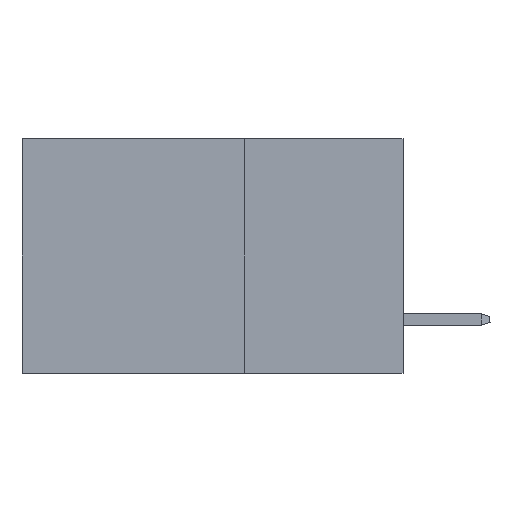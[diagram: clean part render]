
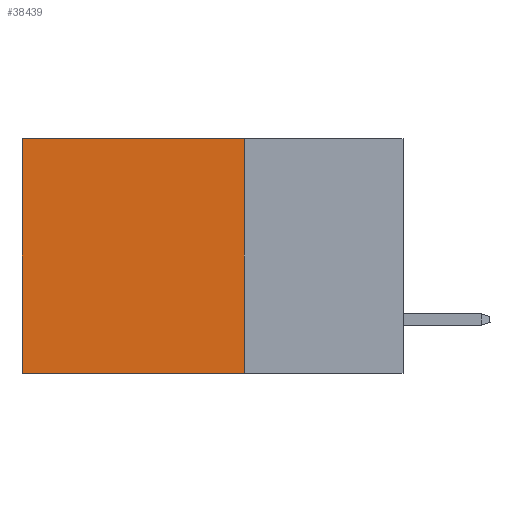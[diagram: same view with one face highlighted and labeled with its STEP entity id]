
A CAD part, left-side view. The second image highlights one B-rep face of the part: STEP entity #38439.
In plain terms, the highlighted planar face has unit normal (-1, 0, 0).
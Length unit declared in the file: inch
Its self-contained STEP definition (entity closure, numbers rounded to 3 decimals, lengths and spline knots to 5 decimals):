
#298 = EDGE_CURVE ( 'NONE', #982, #2464, #387, .T. ) ;
#365 = ORIENTED_EDGE ( 'NONE', *, *, #30370, .T. ) ;
#387 = LINE ( 'NONE', #4774, #18558 ) ;
#982 = VERTEX_POINT ( 'NONE', #10057 ) ;
#2464 = VERTEX_POINT ( 'NONE', #10327 ) ;
#2769 = PLANE ( 'NONE',  #32725 ) ;
#4774 = CARTESIAN_POINT ( 'NONE',  ( 0.2875, 0.25, -0.37 ) ) ;
#5797 = EDGE_LOOP ( 'NONE', ( #17149, #30770, #29971, #365 ) ) ;
#7968 = DIRECTION ( 'NONE',  ( 0., 1., 0. ) ) ;
#8990 = VERTEX_POINT ( 'NONE', #40663 ) ;
#10057 = CARTESIAN_POINT ( 'NONE',  ( 0.2875, 0.25, -0.37 ) ) ;
#10327 = CARTESIAN_POINT ( 'NONE',  ( 0.2875, 0.6, -0.37 ) ) ;
#11798 = DIRECTION ( 'NONE',  ( 0., 0., -1. ) ) ;
#12013 = CARTESIAN_POINT ( 'NONE',  ( 0.2875, 0.25, 0. ) ) ;
#12520 = VECTOR ( 'NONE', #30075, 39.37008 ) ;
#17149 = ORIENTED_EDGE ( 'NONE', *, *, #37518, .T. ) ;
#18558 = VECTOR ( 'NONE', #7968, 39.37008 ) ;
#18881 = CARTESIAN_POINT ( 'NONE',  ( 0.2875, 0.6, 0. ) ) ;
#19336 = LINE ( 'NONE', #12013, #43485 ) ;
#19442 = EDGE_CURVE ( 'NONE', #45630, #982, #19336, .T. ) ;
#22244 = CARTESIAN_POINT ( 'NONE',  ( 0.2875, 0.25, 0. ) ) ;
#26470 = LINE ( 'NONE', #18881, #32688 ) ;
#28960 = CARTESIAN_POINT ( 'NONE',  ( 0.2875, 0.25, 0. ) ) ;
#29971 = ORIENTED_EDGE ( 'NONE', *, *, #19442, .F. ) ;
#30075 = DIRECTION ( 'NONE',  ( 0., 1., 0. ) ) ;
#30370 = EDGE_CURVE ( 'NONE', #45630, #8990, #37413, .T. ) ;
#30770 = ORIENTED_EDGE ( 'NONE', *, *, #298, .F. ) ;
#30841 = DIRECTION ( 'NONE',  ( 0., 0., -1. ) ) ;
#31642 = CARTESIAN_POINT ( 'NONE',  ( 0.2875, 0.25, 0. ) ) ;
#32688 = VECTOR ( 'NONE', #11798, 39.37008 ) ;
#32725 = AXIS2_PLACEMENT_3D ( 'NONE', #31642, #43374, #39706 ) ;
#37413 = LINE ( 'NONE', #22244, #12520 ) ;
#37518 = EDGE_CURVE ( 'NONE', #8990, #2464, #26470, .T. ) ;
#38439 = ADVANCED_FACE ( 'NONE', ( #43607 ), #2769, .F. ) ;
#39706 = DIRECTION ( 'NONE',  ( 0., 0., -1. ) ) ;
#40663 = CARTESIAN_POINT ( 'NONE',  ( 0.2875, 0.6, 0. ) ) ;
#43374 = DIRECTION ( 'NONE',  ( 1., 0., 0. ) ) ;
#43485 = VECTOR ( 'NONE', #30841, 39.37008 ) ;
#43607 = FACE_OUTER_BOUND ( 'NONE', #5797, .T. ) ;
#45630 = VERTEX_POINT ( 'NONE', #28960 ) ;
